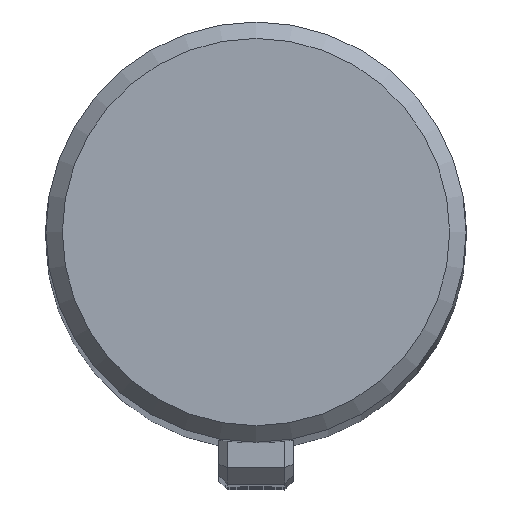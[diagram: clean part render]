
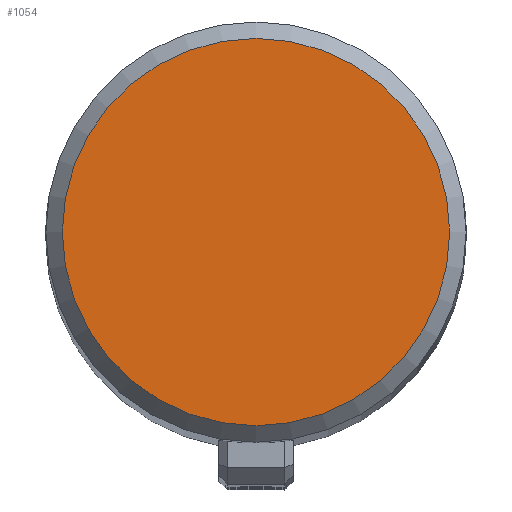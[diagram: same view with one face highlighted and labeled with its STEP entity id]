
A CAD part, top view. The second image highlights one B-rep face of the part: STEP entity #1054.
In plain terms, the highlighted planar face has unit normal (0, 0, 1).
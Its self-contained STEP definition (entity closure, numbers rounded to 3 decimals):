
#42=PLANE('',#1139);
#103=FACE_OUTER_BOUND('',#168,.T.);
#168=EDGE_LOOP('',(#725));
#392=CIRCLE('',#1131,11.75);
#438=VERTEX_POINT('',#1545);
#540=EDGE_CURVE('',#438,#438,#392,.T.);
#725=ORIENTED_EDGE('',*,*,#540,.F.);
#1054=ADVANCED_FACE('',(#103),#42,.F.);
#1131=AXIS2_PLACEMENT_3D('',#1546,#1244,#1245);
#1139=AXIS2_PLACEMENT_3D('',#1635,#1265,#1266);
#1244=DIRECTION('center_axis',(0.,0.,-1.));
#1245=DIRECTION('ref_axis',(1.,0.,0.));
#1265=DIRECTION('center_axis',(0.,0.,-1.));
#1266=DIRECTION('ref_axis',(1.,0.,0.));
#1545=CARTESIAN_POINT('',(-11.75,18.542,-23.142));
#1546=CARTESIAN_POINT('Origin',(0.,18.542,-23.142));
#1635=CARTESIAN_POINT('Origin',(0.,18.542,-23.142));
